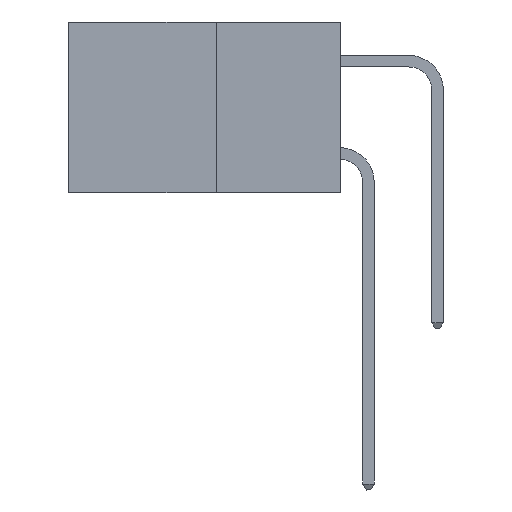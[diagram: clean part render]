
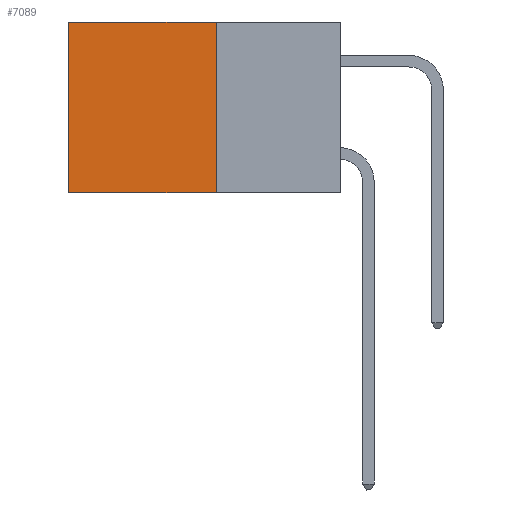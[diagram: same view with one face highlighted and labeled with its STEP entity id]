
A CAD part, left-side view. The second image highlights one B-rep face of the part: STEP entity #7089.
In plain terms, the highlighted planar face has unit normal (-1, 0, 0).
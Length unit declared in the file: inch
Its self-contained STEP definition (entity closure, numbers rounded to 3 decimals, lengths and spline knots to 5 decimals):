
#109 = EDGE_CURVE ( 'NONE', #7282, #7811, #2208, .T. ) ;
#648 = DIRECTION ( 'NONE',  ( 0., 0., -1. ) ) ;
#696 = FACE_OUTER_BOUND ( 'NONE', #8957, .T. ) ;
#879 = PLANE ( 'NONE',  #6248 ) ;
#1028 = LINE ( 'NONE', #7746, #2767 ) ;
#1057 = CARTESIAN_POINT ( 'NONE',  ( 0.277, 0.59, -0.37 ) ) ;
#1140 = DIRECTION ( 'NONE',  ( 0., 1., 0. ) ) ;
#1409 = CARTESIAN_POINT ( 'NONE',  ( 0.277, 0.27, -0.37 ) ) ;
#1489 = DIRECTION ( 'NONE',  ( 0., 0., -1. ) ) ;
#1941 = VECTOR ( 'NONE', #1140, 39.37008 ) ;
#2208 = LINE ( 'NONE', #10821, #1941 ) ;
#2350 = ORIENTED_EDGE ( 'NONE', *, *, #2653, .T. ) ;
#2362 = ORIENTED_EDGE ( 'NONE', *, *, #9893, .F. ) ;
#2371 = ORIENTED_EDGE ( 'NONE', *, *, #5794, .F. ) ;
#2381 = ORIENTED_EDGE ( 'NONE', *, *, #109, .T. ) ;
#2595 = DIRECTION ( 'NONE',  ( 0., 0., -1. ) ) ;
#2653 = EDGE_CURVE ( 'NONE', #7811, #4266, #10193, .T. ) ;
#2767 = VECTOR ( 'NONE', #5148, 39.37008 ) ;
#3714 = CARTESIAN_POINT ( 'NONE',  ( 0.277, 0.27, 0. ) ) ;
#4266 = VERTEX_POINT ( 'NONE', #5888 ) ;
#4857 = LINE ( 'NONE', #1409, #7192 ) ;
#5049 = VERTEX_POINT ( 'NONE', #7428 ) ;
#5078 = VECTOR ( 'NONE', #648, 39.37008 ) ;
#5148 = DIRECTION ( 'NONE',  ( 0., 1., 0. ) ) ;
#5331 = CARTESIAN_POINT ( 'NONE',  ( 0.277, 0.59, 0. ) ) ;
#5794 = EDGE_CURVE ( 'NONE', #7282, #5049, #4857, .T. ) ;
#5888 = CARTESIAN_POINT ( 'NONE',  ( 0.277, 0.59, -0.37 ) ) ;
#6248 = AXIS2_PLACEMENT_3D ( 'NONE', #7025, #7888, #2595 ) ;
#7025 = CARTESIAN_POINT ( 'NONE',  ( 0.277, 0.27, -0.37 ) ) ;
#7089 = ADVANCED_FACE ( 'NONE', ( #696 ), #879, .F. ) ;
#7192 = VECTOR ( 'NONE', #1489, 39.37008 ) ;
#7282 = VERTEX_POINT ( 'NONE', #3714 ) ;
#7428 = CARTESIAN_POINT ( 'NONE',  ( 0.277, 0.27, -0.37 ) ) ;
#7746 = CARTESIAN_POINT ( 'NONE',  ( 0.277, 0.27, -0.37 ) ) ;
#7811 = VERTEX_POINT ( 'NONE', #5331 ) ;
#7888 = DIRECTION ( 'NONE',  ( 1., 0., 0. ) ) ;
#8957 = EDGE_LOOP ( 'NONE', ( #2350, #2362, #2371, #2381 ) ) ;
#9893 = EDGE_CURVE ( 'NONE', #5049, #4266, #1028, .T. ) ;
#10193 = LINE ( 'NONE', #1057, #5078 ) ;
#10821 = CARTESIAN_POINT ( 'NONE',  ( 0.277, 0.27, 0. ) ) ;
